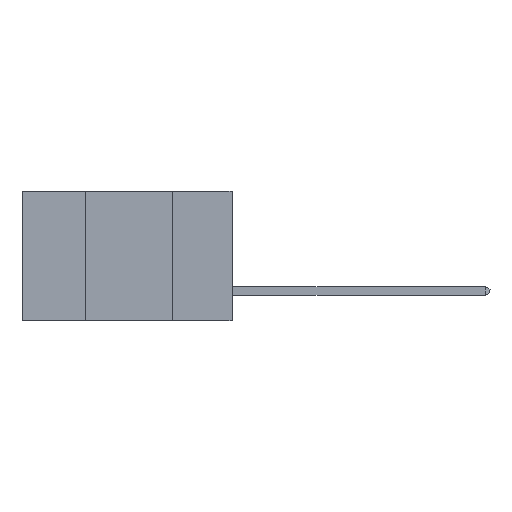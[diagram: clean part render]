
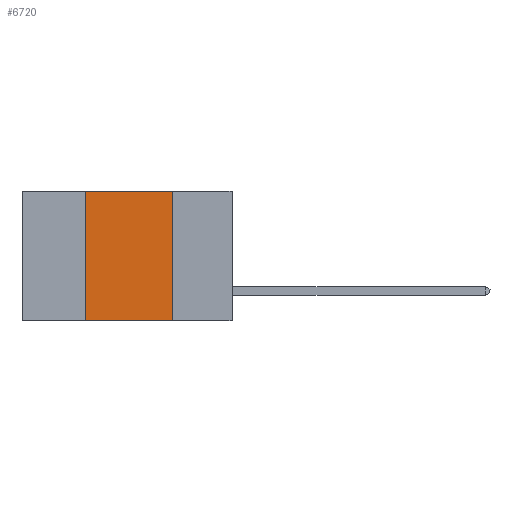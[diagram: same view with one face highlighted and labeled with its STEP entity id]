
A CAD part, left-side view. The second image highlights one B-rep face of the part: STEP entity #6720.
In plain terms, the highlighted planar face has unit normal (-1, 0, 0).
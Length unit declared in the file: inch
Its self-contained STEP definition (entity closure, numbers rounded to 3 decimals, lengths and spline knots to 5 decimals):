
#446 = VERTEX_POINT ( 'NONE', #9233 ) ;
#685 = DIRECTION ( 'NONE',  ( 0., -1., 0. ) ) ;
#1094 = LINE ( 'NONE', #4714, #5801 ) ;
#1767 = ORIENTED_EDGE ( 'NONE', *, *, #2735, .T. ) ;
#1834 = DIRECTION ( 'NONE',  ( 0., 0., -1. ) ) ;
#2562 = AXIS2_PLACEMENT_3D ( 'NONE', #2639, #6539, #9452 ) ;
#2639 = CARTESIAN_POINT ( 'NONE',  ( 0., 0.6, 0. ) ) ;
#2735 = EDGE_CURVE ( 'NONE', #446, #8246, #1094, .T. ) ;
#4714 = CARTESIAN_POINT ( 'NONE',  ( 0., 0.6, -0.37 ) ) ;
#5024 = ORIENTED_EDGE ( 'NONE', *, *, #11976, .F. ) ;
#5428 = CARTESIAN_POINT ( 'NONE',  ( 0., 0.6, 0. ) ) ;
#5766 = VECTOR ( 'NONE', #685, 39.37008 ) ;
#5801 = VECTOR ( 'NONE', #12238, 39.37008 ) ;
#6185 = EDGE_LOOP ( 'NONE', ( #8002, #5024, #10525, #1767 ) ) ;
#6493 = VECTOR ( 'NONE', #12165, 39.37008 ) ;
#6539 = DIRECTION ( 'NONE',  ( 1., 0., 0. ) ) ;
#6650 = EDGE_CURVE ( 'NONE', #446, #8360, #9043, .T. ) ;
#6720 = ADVANCED_FACE ( 'NONE', ( #8896 ), #7696, .F. ) ;
#7253 = CARTESIAN_POINT ( 'NONE',  ( 0., 0.42, 0. ) ) ;
#7559 = CARTESIAN_POINT ( 'NONE',  ( 0., 0.17, 0. ) ) ;
#7696 = PLANE ( 'NONE',  #2562 ) ;
#8002 = ORIENTED_EDGE ( 'NONE', *, *, #10382, .F. ) ;
#8031 = CARTESIAN_POINT ( 'NONE',  ( 0., 0.17, 0. ) ) ;
#8135 = CARTESIAN_POINT ( 'NONE',  ( 0., 0.17, -0.37 ) ) ;
#8246 = VERTEX_POINT ( 'NONE', #8135 ) ;
#8360 = VERTEX_POINT ( 'NONE', #10312 ) ;
#8654 = LINE ( 'NONE', #7559, #11537 ) ;
#8896 = FACE_OUTER_BOUND ( 'NONE', #6185, .T. ) ;
#9043 = LINE ( 'NONE', #7253, #6493 ) ;
#9233 = CARTESIAN_POINT ( 'NONE',  ( 0., 0.42, -0.37 ) ) ;
#9452 = DIRECTION ( 'NONE',  ( 0., 0., -1. ) ) ;
#10312 = CARTESIAN_POINT ( 'NONE',  ( 0., 0.42, 0. ) ) ;
#10382 = EDGE_CURVE ( 'NONE', #11304, #8246, #8654, .T. ) ;
#10525 = ORIENTED_EDGE ( 'NONE', *, *, #6650, .F. ) ;
#10893 = LINE ( 'NONE', #5428, #5766 ) ;
#11304 = VERTEX_POINT ( 'NONE', #8031 ) ;
#11537 = VECTOR ( 'NONE', #1834, 39.37008 ) ;
#11976 = EDGE_CURVE ( 'NONE', #8360, #11304, #10893, .T. ) ;
#12165 = DIRECTION ( 'NONE',  ( 0., 0., 1. ) ) ;
#12238 = DIRECTION ( 'NONE',  ( 0., -1., 0. ) ) ;
